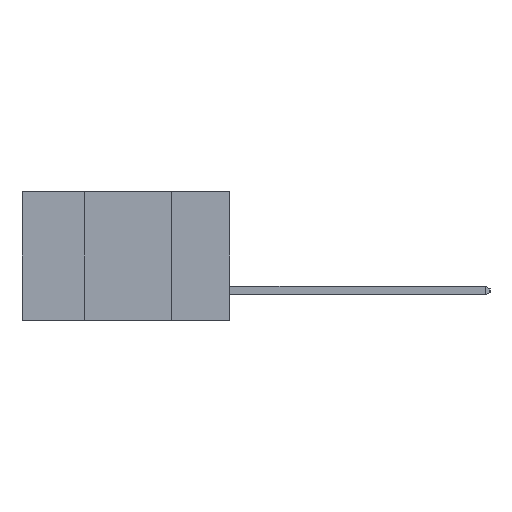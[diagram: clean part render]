
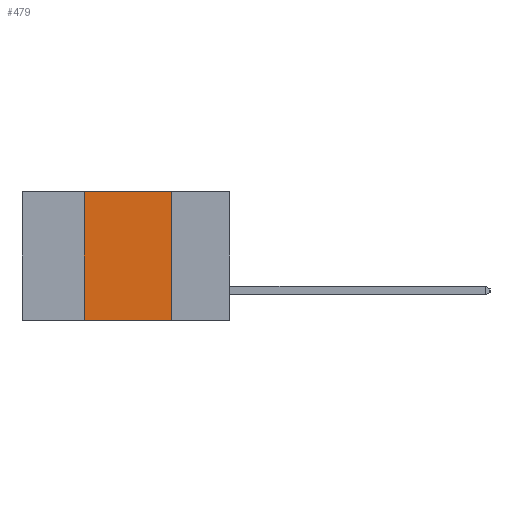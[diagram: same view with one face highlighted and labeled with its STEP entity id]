
A CAD part, left-side view. The second image highlights one B-rep face of the part: STEP entity #479.
In plain terms, the highlighted planar face has unit normal (-1, 0, 0).
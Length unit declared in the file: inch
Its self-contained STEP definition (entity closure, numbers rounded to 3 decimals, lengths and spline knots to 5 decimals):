
#239 = AXIS2_PLACEMENT_3D ( 'NONE', #15583, #15439, #14361 ) ;
#479 = ADVANCED_FACE ( 'NONE', ( #21885 ), #17645, .F. ) ;
#1068 = VECTOR ( 'NONE', #18455, 39.37008 ) ;
#2358 = VECTOR ( 'NONE', #5973, 39.37008 ) ;
#3783 = EDGE_CURVE ( 'NONE', #22286, #21252, #22008, .T. ) ;
#4024 = CARTESIAN_POINT ( 'NONE',  ( 0., 0.6, 0. ) ) ;
#4135 = DIRECTION ( 'NONE',  ( 0., 0., -1. ) ) ;
#4762 = ORIENTED_EDGE ( 'NONE', *, *, #17418, .F. ) ;
#5471 = DIRECTION ( 'NONE',  ( 0., 0., 1. ) ) ;
#5973 = DIRECTION ( 'NONE',  ( 0., -1., 0. ) ) ;
#6307 = ORIENTED_EDGE ( 'NONE', *, *, #3783, .T. ) ;
#10574 = VERTEX_POINT ( 'NONE', #15273 ) ;
#10579 = EDGE_LOOP ( 'NONE', ( #4762, #25273, #21405, #6307 ) ) ;
#12002 = CARTESIAN_POINT ( 'NONE',  ( 0., 0.42, -0.37 ) ) ;
#14361 = DIRECTION ( 'NONE',  ( 0., 0., -1. ) ) ;
#15273 = CARTESIAN_POINT ( 'NONE',  ( 0., 0.42, 0. ) ) ;
#15439 = DIRECTION ( 'NONE',  ( 1., 0., 0. ) ) ;
#15583 = CARTESIAN_POINT ( 'NONE',  ( 0., 0.6, 0. ) ) ;
#16617 = VERTEX_POINT ( 'NONE', #19612 ) ;
#17418 = EDGE_CURVE ( 'NONE', #16617, #21252, #24808, .T. ) ;
#17645 = PLANE ( 'NONE',  #239 ) ;
#17886 = LINE ( 'NONE', #24973, #22490 ) ;
#18025 = LINE ( 'NONE', #4024, #2358 ) ;
#18340 = CARTESIAN_POINT ( 'NONE',  ( 0., 0.6, -0.37 ) ) ;
#18455 = DIRECTION ( 'NONE',  ( 0., -1., 0. ) ) ;
#19057 = VECTOR ( 'NONE', #4135, 39.37008 ) ;
#19612 = CARTESIAN_POINT ( 'NONE',  ( 0., 0.17, 0. ) ) ;
#19832 = CARTESIAN_POINT ( 'NONE',  ( 0., 0.17, -0.37 ) ) ;
#20062 = EDGE_CURVE ( 'NONE', #10574, #16617, #18025, .T. ) ;
#20090 = CARTESIAN_POINT ( 'NONE',  ( 0., 0.17, -0.37 ) ) ;
#21252 = VERTEX_POINT ( 'NONE', #20090 ) ;
#21405 = ORIENTED_EDGE ( 'NONE', *, *, #23949, .F. ) ;
#21885 = FACE_OUTER_BOUND ( 'NONE', #10579, .T. ) ;
#22008 = LINE ( 'NONE', #18340, #1068 ) ;
#22286 = VERTEX_POINT ( 'NONE', #12002 ) ;
#22490 = VECTOR ( 'NONE', #5471, 39.37008 ) ;
#23949 = EDGE_CURVE ( 'NONE', #22286, #10574, #17886, .T. ) ;
#24808 = LINE ( 'NONE', #19832, #19057 ) ;
#24973 = CARTESIAN_POINT ( 'NONE',  ( 0., 0.42, -0.37 ) ) ;
#25273 = ORIENTED_EDGE ( 'NONE', *, *, #20062, .F. ) ;
